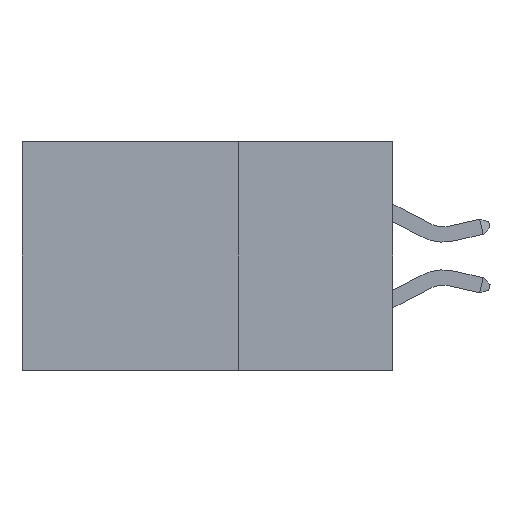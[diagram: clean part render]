
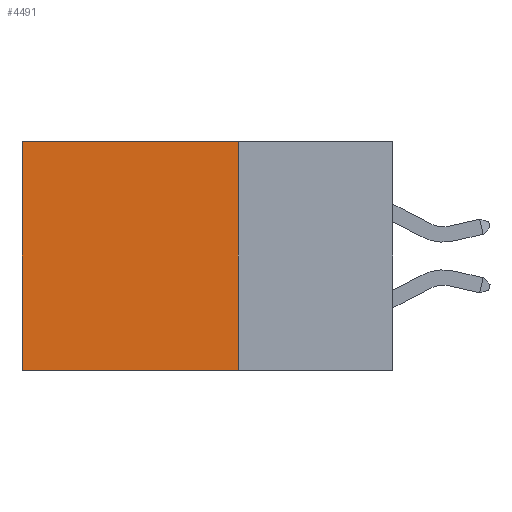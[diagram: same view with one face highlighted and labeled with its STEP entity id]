
A CAD part, left-side view. The second image highlights one B-rep face of the part: STEP entity #4491.
In plain terms, the highlighted planar face has unit normal (-1, 0, 0).
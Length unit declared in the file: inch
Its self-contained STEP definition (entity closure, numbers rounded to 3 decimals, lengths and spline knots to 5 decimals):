
#769 = VERTEX_POINT ( 'NONE', #2696 ) ;
#1550 = VECTOR ( 'NONE', #21474, 39.37008 ) ;
#1817 = VECTOR ( 'NONE', #6088, 39.37008 ) ;
#2577 = LINE ( 'NONE', #16517, #21718 ) ;
#2696 = CARTESIAN_POINT ( 'NONE',  ( 0.2875, 0.25, 0. ) ) ;
#3020 = EDGE_CURVE ( 'NONE', #769, #21773, #13101, .T. ) ;
#3402 = DIRECTION ( 'NONE',  ( 1., 0., 0. ) ) ;
#3708 = ORIENTED_EDGE ( 'NONE', *, *, #7865, .F. ) ;
#4491 = ADVANCED_FACE ( 'NONE', ( #12517 ), #17962, .F. ) ;
#4546 = DIRECTION ( 'NONE',  ( 0., 1., 0. ) ) ;
#4858 = AXIS2_PLACEMENT_3D ( 'NONE', #23879, #3402, #15035 ) ;
#5522 = EDGE_CURVE ( 'NONE', #6646, #13623, #19431, .T. ) ;
#5551 = DIRECTION ( 'NONE',  ( 0., 1., 0. ) ) ;
#6088 = DIRECTION ( 'NONE',  ( 0., 0., -1. ) ) ;
#6646 = VERTEX_POINT ( 'NONE', #15649 ) ;
#7865 = EDGE_CURVE ( 'NONE', #21773, #13623, #19004, .T. ) ;
#8106 = ORIENTED_EDGE ( 'NONE', *, *, #10950, .T. ) ;
#9834 = CARTESIAN_POINT ( 'NONE',  ( 0.2875, 0.6, 0. ) ) ;
#10055 = CARTESIAN_POINT ( 'NONE',  ( 0.2875, 0.25, 0. ) ) ;
#10191 = ORIENTED_EDGE ( 'NONE', *, *, #5522, .T. ) ;
#10631 = VECTOR ( 'NONE', #4546, 39.37008 ) ;
#10950 = EDGE_CURVE ( 'NONE', #769, #6646, #2577, .T. ) ;
#12517 = FACE_OUTER_BOUND ( 'NONE', #20291, .T. ) ;
#13101 = LINE ( 'NONE', #10055, #1550 ) ;
#13623 = VERTEX_POINT ( 'NONE', #20219 ) ;
#14615 = CARTESIAN_POINT ( 'NONE',  ( 0.2875, 0.25, -0.37 ) ) ;
#15035 = DIRECTION ( 'NONE',  ( 0., 0., -1. ) ) ;
#15649 = CARTESIAN_POINT ( 'NONE',  ( 0.2875, 0.6, 0. ) ) ;
#16517 = CARTESIAN_POINT ( 'NONE',  ( 0.2875, 0.25, 0. ) ) ;
#17962 = PLANE ( 'NONE',  #4858 ) ;
#19004 = LINE ( 'NONE', #19534, #10631 ) ;
#19431 = LINE ( 'NONE', #9834, #1817 ) ;
#19534 = CARTESIAN_POINT ( 'NONE',  ( 0.2875, 0.25, -0.37 ) ) ;
#20219 = CARTESIAN_POINT ( 'NONE',  ( 0.2875, 0.6, -0.37 ) ) ;
#20291 = EDGE_LOOP ( 'NONE', ( #10191, #3708, #23659, #8106 ) ) ;
#21474 = DIRECTION ( 'NONE',  ( 0., 0., -1. ) ) ;
#21718 = VECTOR ( 'NONE', #5551, 39.37008 ) ;
#21773 = VERTEX_POINT ( 'NONE', #14615 ) ;
#23659 = ORIENTED_EDGE ( 'NONE', *, *, #3020, .F. ) ;
#23879 = CARTESIAN_POINT ( 'NONE',  ( 0.2875, 0.25, 0. ) ) ;
